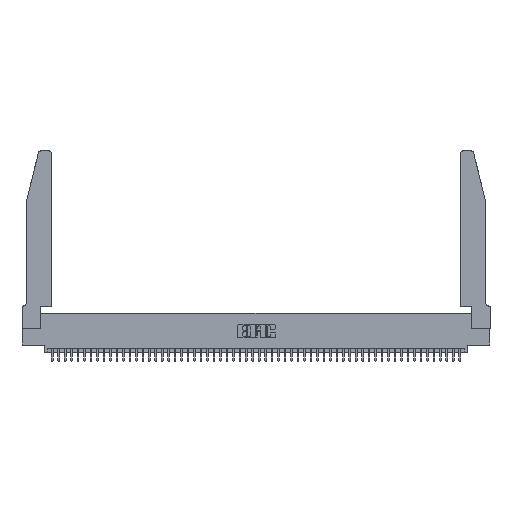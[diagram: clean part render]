
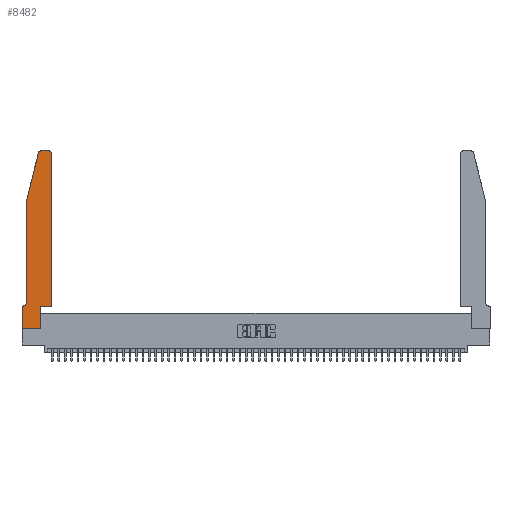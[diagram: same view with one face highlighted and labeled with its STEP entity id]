
A CAD part, top view. The second image highlights one B-rep face of the part: STEP entity #8482.
In plain terms, the highlighted planar face has unit normal (0, 0, 1).
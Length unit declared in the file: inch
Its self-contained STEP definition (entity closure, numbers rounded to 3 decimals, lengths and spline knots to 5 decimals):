
#738 = EDGE_CURVE ( 'NONE', #10546, #23717, #40464, .T. ) ;
#1176 = VERTEX_POINT ( 'NONE', #50721 ) ;
#2016 = VERTEX_POINT ( 'NONE', #29142 ) ;
#2244 = LINE ( 'NONE', #16130, #14243 ) ;
#2398 = DIRECTION ( 'NONE',  ( 1., 0., 0. ) ) ;
#2808 = EDGE_CURVE ( 'NONE', #46168, #33491, #47085, .T. ) ;
#2941 = VERTEX_POINT ( 'NONE', #23054 ) ;
#3090 = EDGE_CURVE ( 'NONE', #2016, #11192, #11803, .T. ) ;
#3146 = DIRECTION ( 'NONE',  ( 1., 0., 0. ) ) ;
#3775 = VECTOR ( 'NONE', #50736, 39.37008 ) ;
#3917 = CIRCLE ( 'NONE', #51193, 0.07 ) ;
#4228 = VECTOR ( 'NONE', #14237, 39.37008 ) ;
#4307 = ORIENTED_EDGE ( 'NONE', *, *, #738, .T. ) ;
#4371 = EDGE_CURVE ( 'NONE', #2941, #33113, #37631, .T. ) ;
#4463 = DIRECTION ( 'NONE',  ( 0., 0., 1. ) ) ;
#4660 = EDGE_CURVE ( 'NONE', #23717, #4954, #2244, .T. ) ;
#4739 = DIRECTION ( 'NONE',  ( 0., 0., -1. ) ) ;
#4954 = VERTEX_POINT ( 'NONE', #27046 ) ;
#4984 = ORIENTED_EDGE ( 'NONE', *, *, #13214, .T. ) ;
#5868 = CARTESIAN_POINT ( 'NONE',  ( 0.2865, 0., 0.37 ) ) ;
#6574 = EDGE_CURVE ( 'NONE', #42841, #1176, #38101, .T. ) ;
#7251 = EDGE_CURVE ( 'NONE', #33491, #2016, #3917, .T. ) ;
#8417 = EDGE_CURVE ( 'NONE', #18321, #42841, #17090, .T. ) ;
#8482 = ADVANCED_FACE ( 'NONE', ( #51055 ), #15002, .T. ) ;
#8530 = DIRECTION ( 'NONE',  ( 0., 1., 0. ) ) ;
#8578 = ORIENTED_EDGE ( 'NONE', *, *, #8417, .T. ) ;
#9398 = ORIENTED_EDGE ( 'NONE', *, *, #2808, .T. ) ;
#9855 = VECTOR ( 'NONE', #23910, 39.37008 ) ;
#10546 = VERTEX_POINT ( 'NONE', #11640 ) ;
#11192 = VERTEX_POINT ( 'NONE', #18298 ) ;
#11640 = CARTESIAN_POINT ( 'NONE',  ( 0., 0., 0.37 ) ) ;
#11803 = LINE ( 'NONE', #40284, #21948 ) ;
#12424 = ORIENTED_EDGE ( 'NONE', *, *, #3090, .T. ) ;
#13129 = DIRECTION ( 'NONE',  ( 1., 0., 0. ) ) ;
#13214 = EDGE_CURVE ( 'NONE', #4954, #2941, #38405, .T. ) ;
#13957 = CARTESIAN_POINT ( 'NONE',  ( 0.2605, 2.75, 0.37 ) ) ;
#14237 = DIRECTION ( 'NONE',  ( 0., -1., 0. ) ) ;
#14243 = VECTOR ( 'NONE', #8530, 39.37008 ) ;
#15002 = PLANE ( 'NONE',  #37442 ) ;
#15254 = LINE ( 'NONE', #19864, #44854 ) ;
#16130 = CARTESIAN_POINT ( 'NONE',  ( 0.2865, 0.35, 0.37 ) ) ;
#17090 = LINE ( 'NONE', #13957, #3775 ) ;
#18298 = CARTESIAN_POINT ( 'NONE',  ( 0., 0.35, 0.37 ) ) ;
#18321 = VERTEX_POINT ( 'NONE', #42665 ) ;
#19061 = DIRECTION ( 'NONE',  ( 0., 0., 1. ) ) ;
#19864 = CARTESIAN_POINT ( 'NONE',  ( 0.0755, 2., 0.37 ) ) ;
#21596 = ORIENTED_EDGE ( 'NONE', *, *, #30920, .T. ) ;
#21948 = VECTOR ( 'NONE', #23919, 39.37008 ) ;
#22033 = DIRECTION ( 'NONE',  ( 0., 0., 1. ) ) ;
#23054 = CARTESIAN_POINT ( 'NONE',  ( 0.4505, 0.35, 0.37 ) ) ;
#23395 = CARTESIAN_POINT ( 'NONE',  ( 0.4505, 0.35, 0.37 ) ) ;
#23717 = VERTEX_POINT ( 'NONE', #5868 ) ;
#23753 = CARTESIAN_POINT ( 'NONE',  ( 0., 0., 0.37 ) ) ;
#23910 = DIRECTION ( 'NONE',  ( 0., 1., 0. ) ) ;
#23919 = DIRECTION ( 'NONE',  ( -1., 0., 0. ) ) ;
#24692 = ORIENTED_EDGE ( 'NONE', *, *, #7251, .T. ) ;
#25404 = CARTESIAN_POINT ( 'NONE',  ( 0.4505, 2.72, 0.37 ) ) ;
#26420 = CARTESIAN_POINT ( 'NONE',  ( 0.4205, 2.72, 0.37 ) ) ;
#26423 = CARTESIAN_POINT ( 'NONE',  ( 0.0755, 2., 0.37 ) ) ;
#27046 = CARTESIAN_POINT ( 'NONE',  ( 0.2865, 0.35, 0.37 ) ) ;
#28109 = CARTESIAN_POINT ( 'NONE',  ( 0., 0., 0.37 ) ) ;
#28909 = ORIENTED_EDGE ( 'NONE', *, *, #29144, .T. ) ;
#29142 = CARTESIAN_POINT ( 'NONE',  ( 0.0055, 0.35, 0.37 ) ) ;
#29144 = EDGE_CURVE ( 'NONE', #11192, #10546, #34944, .T. ) ;
#29785 = VECTOR ( 'NONE', #31634, 39.37008 ) ;
#29968 = DIRECTION ( 'NONE',  ( 1., 0., 0. ) ) ;
#30920 = EDGE_CURVE ( 'NONE', #33113, #18321, #44249, .T. ) ;
#31290 = EDGE_CURVE ( 'NONE', #1176, #46168, #15254, .T. ) ;
#31634 = DIRECTION ( 'NONE',  ( 1., 0., 0. ) ) ;
#31877 = DIRECTION ( 'NONE',  ( 0., -1., 0. ) ) ;
#32204 = CARTESIAN_POINT ( 'NONE',  ( 0.4505, 0.35, 0.37 ) ) ;
#33113 = VERTEX_POINT ( 'NONE', #25404 ) ;
#33491 = VERTEX_POINT ( 'NONE', #39256 ) ;
#34944 = LINE ( 'NONE', #23753, #38114 ) ;
#35491 = EDGE_LOOP ( 'NONE', ( #8578, #46198, #42458, #9398, #24692, #12424, #28909, #4307, #40889, #4984, #49149, #21596 ) ) ;
#37220 = DIRECTION ( 'NONE',  ( -1., 0., 0. ) ) ;
#37442 = AXIS2_PLACEMENT_3D ( 'NONE', #43164, #19061, #3146 ) ;
#37631 = LINE ( 'NONE', #32204, #9855 ) ;
#38101 = CIRCLE ( 'NONE', #48799, 0.03 ) ;
#38114 = VECTOR ( 'NONE', #31877, 39.37008 ) ;
#38405 = LINE ( 'NONE', #23395, #49098 ) ;
#39256 = CARTESIAN_POINT ( 'NONE',  ( 0.0755, 0.42, 0.37 ) ) ;
#40284 = CARTESIAN_POINT ( 'NONE',  ( 0.0755, 0.35, 0.37 ) ) ;
#40464 = LINE ( 'NONE', #28109, #29785 ) ;
#40794 = CARTESIAN_POINT ( 'NONE',  ( 0.284, 2.72, 0.37 ) ) ;
#40889 = ORIENTED_EDGE ( 'NONE', *, *, #4660, .T. ) ;
#42458 = ORIENTED_EDGE ( 'NONE', *, *, #31290, .T. ) ;
#42614 = CARTESIAN_POINT ( 'NONE',  ( 0.0755, 2., 0.37 ) ) ;
#42665 = CARTESIAN_POINT ( 'NONE',  ( 0.4205, 2.75, 0.37 ) ) ;
#42841 = VERTEX_POINT ( 'NONE', #45909 ) ;
#43164 = CARTESIAN_POINT ( 'NONE',  ( 0., 0.35, 0.37 ) ) ;
#43171 = AXIS2_PLACEMENT_3D ( 'NONE', #26420, #22033, #29968 ) ;
#44249 = CIRCLE ( 'NONE', #43171, 0.03 ) ;
#44854 = VECTOR ( 'NONE', #51546, 39.37008 ) ;
#45445 = CARTESIAN_POINT ( 'NONE',  ( 0.0055, 0.42, 0.37 ) ) ;
#45909 = CARTESIAN_POINT ( 'NONE',  ( 0.284, 2.75, 0.37 ) ) ;
#46168 = VERTEX_POINT ( 'NONE', #42614 ) ;
#46198 = ORIENTED_EDGE ( 'NONE', *, *, #6574, .T. ) ;
#47085 = LINE ( 'NONE', #26423, #4228 ) ;
#48799 = AXIS2_PLACEMENT_3D ( 'NONE', #40794, #4463, #13129 ) ;
#49098 = VECTOR ( 'NONE', #2398, 39.37008 ) ;
#49149 = ORIENTED_EDGE ( 'NONE', *, *, #4371, .T. ) ;
#50721 = CARTESIAN_POINT ( 'NONE',  ( 0.25487, 2.72718, 0.37 ) ) ;
#50736 = DIRECTION ( 'NONE',  ( -1., 0., 0. ) ) ;
#51055 = FACE_OUTER_BOUND ( 'NONE', #35491, .T. ) ;
#51193 = AXIS2_PLACEMENT_3D ( 'NONE', #45445, #4739, #37220 ) ;
#51546 = DIRECTION ( 'NONE',  ( -0.239, -0.971, 0. ) ) ;
